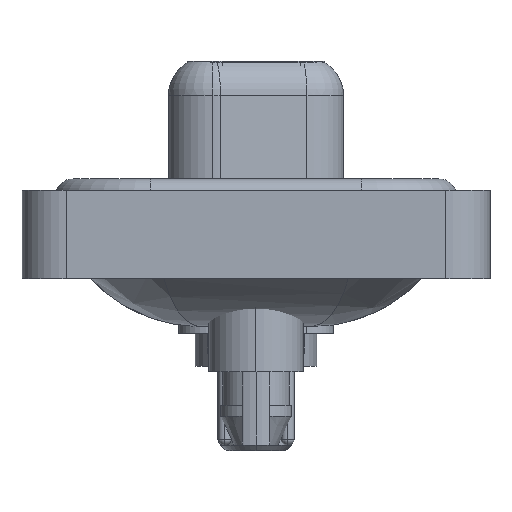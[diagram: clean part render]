
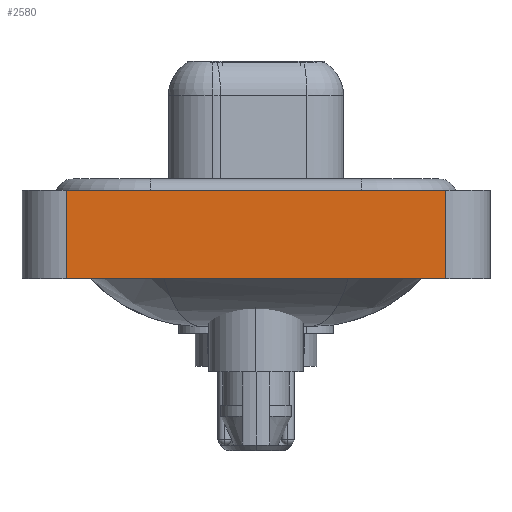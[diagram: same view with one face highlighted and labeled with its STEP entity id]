
A CAD part, left-side view. The second image highlights one B-rep face of the part: STEP entity #2580.
In plain terms, the highlighted planar face has unit normal (-1, 0, 0).
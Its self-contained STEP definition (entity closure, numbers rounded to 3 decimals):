
#247 = CARTESIAN_POINT ( 'NONE',  ( -7.25, -8.55, -3.6 ) ) ;
#312 = DIRECTION ( 'NONE',  ( 0., -1., 0. ) ) ;
#423 = VECTOR ( 'NONE', #5411, 1000. ) ;
#1763 = EDGE_CURVE ( 'NONE', #5400, #8697, #17380, .T. ) ;
#1825 = LINE ( 'NONE', #6009, #17458 ) ;
#1990 = LINE ( 'NONE', #8328, #423 ) ;
#2580 = ADVANCED_FACE ( 'NONE', ( #5038 ), #15943, .T. ) ;
#3173 = LINE ( 'NONE', #9501, #15175 ) ;
#3335 = ORIENTED_EDGE ( 'NONE', *, *, #5585, .F. ) ;
#3746 = CARTESIAN_POINT ( 'NONE',  ( -7.25, 8.55, -3.6 ) ) ;
#5038 = FACE_OUTER_BOUND ( 'NONE', #17999, .T. ) ;
#5109 = VERTEX_POINT ( 'NONE', #10308 ) ;
#5400 = VERTEX_POINT ( 'NONE', #3746 ) ;
#5411 = DIRECTION ( 'NONE',  ( 0., 0., 1. ) ) ;
#5585 = EDGE_CURVE ( 'NONE', #6593, #5109, #1825, .T. ) ;
#6009 = CARTESIAN_POINT ( 'NONE',  ( -7.25, -8.55, 0.4 ) ) ;
#6132 = EDGE_CURVE ( 'NONE', #5400, #6593, #3173, .T. ) ;
#6490 = DIRECTION ( 'NONE',  ( -1., 0., 0. ) ) ;
#6593 = VERTEX_POINT ( 'NONE', #12891 ) ;
#7174 = ORIENTED_EDGE ( 'NONE', *, *, #1763, .T. ) ;
#7851 = ORIENTED_EDGE ( 'NONE', *, *, #6132, .F. ) ;
#8050 = CARTESIAN_POINT ( 'NONE',  ( -7.25, -8.55, -3.6 ) ) ;
#8328 = CARTESIAN_POINT ( 'NONE',  ( -7.25, -8.55, -3.6 ) ) ;
#8697 = VERTEX_POINT ( 'NONE', #247 ) ;
#9501 = CARTESIAN_POINT ( 'NONE',  ( -7.25, 8.55, -3.6 ) ) ;
#10308 = CARTESIAN_POINT ( 'NONE',  ( -7.25, -8.55, 0.4 ) ) ;
#10643 = EDGE_CURVE ( 'NONE', #8697, #5109, #1990, .T. ) ;
#11385 = DIRECTION ( 'NONE',  ( 0., -1., 0. ) ) ;
#12484 = ORIENTED_EDGE ( 'NONE', *, *, #10643, .T. ) ;
#12827 = DIRECTION ( 'NONE',  ( 0., 0., 1. ) ) ;
#12891 = CARTESIAN_POINT ( 'NONE',  ( -7.25, 8.55, 0.4 ) ) ;
#13871 = VECTOR ( 'NONE', #312, 1000. ) ;
#14272 = CARTESIAN_POINT ( 'NONE',  ( -7.25, -8.55, -3.6 ) ) ;
#15175 = VECTOR ( 'NONE', #19159, 1000. ) ;
#15943 = PLANE ( 'NONE',  #19574 ) ;
#17380 = LINE ( 'NONE', #14272, #13871 ) ;
#17458 = VECTOR ( 'NONE', #11385, 1000. ) ;
#17999 = EDGE_LOOP ( 'NONE', ( #12484, #3335, #7851, #7174 ) ) ;
#19159 = DIRECTION ( 'NONE',  ( 0., 0., 1. ) ) ;
#19574 = AXIS2_PLACEMENT_3D ( 'NONE', #8050, #6490, #12827 ) ;
